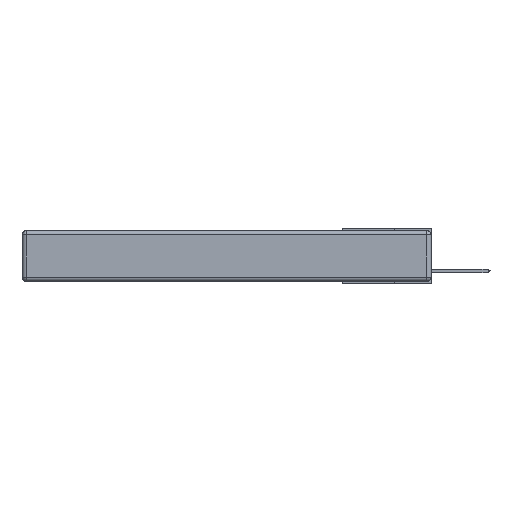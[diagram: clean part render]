
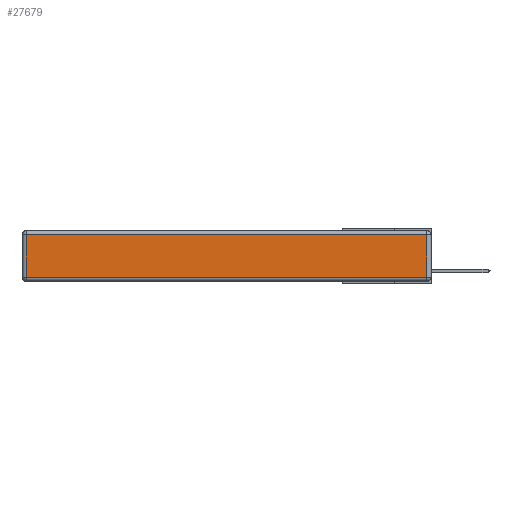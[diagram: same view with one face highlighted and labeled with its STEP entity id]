
A CAD part, left-side view. The second image highlights one B-rep face of the part: STEP entity #27679.
In plain terms, the highlighted planar face has unit normal (-1, 0, 0).
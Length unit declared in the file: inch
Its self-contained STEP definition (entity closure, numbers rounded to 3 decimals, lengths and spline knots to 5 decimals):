
#69 = DIRECTION ( 'NONE',  ( 0., 0., -1. ) ) ;
#555 = VECTOR ( 'NONE', #26867, 39.37008 ) ;
#1219 = VERTEX_POINT ( 'NONE', #25507 ) ;
#1252 = PLANE ( 'NONE',  #25136 ) ;
#1460 = DIRECTION ( 'NONE',  ( -1., 0., 0. ) ) ;
#2239 = VERTEX_POINT ( 'NONE', #18584 ) ;
#2263 = CARTESIAN_POINT ( 'NONE',  ( 0., 0., -0.313 ) ) ;
#2617 = ORIENTED_EDGE ( 'NONE', *, *, #20545, .T. ) ;
#3060 = ORIENTED_EDGE ( 'NONE', *, *, #13140, .T. ) ;
#3183 = CARTESIAN_POINT ( 'NONE',  ( 0., 0., -0.343 ) ) ;
#4995 = CARTESIAN_POINT ( 'NONE',  ( 0., 2.72, -0.343 ) ) ;
#6044 = CARTESIAN_POINT ( 'NONE',  ( 0., 2.75, -0.03 ) ) ;
#6498 = DIRECTION ( 'NONE',  ( 0., 0., 1. ) ) ;
#7588 = EDGE_CURVE ( 'NONE', #2239, #1219, #19691, .T. ) ;
#7644 = DIRECTION ( 'NONE',  ( 0., 0., 1. ) ) ;
#8942 = EDGE_CURVE ( 'NONE', #30396, #2239, #10089, .T. ) ;
#9676 = ORIENTED_EDGE ( 'NONE', *, *, #7588, .T. ) ;
#10089 = LINE ( 'NONE', #2263, #555 ) ;
#12495 = VECTOR ( 'NONE', #69, 39.37008 ) ;
#13140 = EDGE_CURVE ( 'NONE', #24433, #30396, #26180, .T. ) ;
#14855 = CARTESIAN_POINT ( 'NONE',  ( 0., 0.03, -0.343 ) ) ;
#15329 = FACE_OUTER_BOUND ( 'NONE', #15838, .T. ) ;
#15838 = EDGE_LOOP ( 'NONE', ( #23708, #9676, #2617, #3060 ) ) ;
#18584 = CARTESIAN_POINT ( 'NONE',  ( 0., 0.03, -0.313 ) ) ;
#19691 = LINE ( 'NONE', #14855, #20078 ) ;
#20078 = VECTOR ( 'NONE', #7644, 39.37008 ) ;
#20545 = EDGE_CURVE ( 'NONE', #1219, #24433, #22222, .T. ) ;
#21069 = VECTOR ( 'NONE', #21180, 39.37008 ) ;
#21118 = CARTESIAN_POINT ( 'NONE',  ( 0., 2.72, -0.313 ) ) ;
#21180 = DIRECTION ( 'NONE',  ( 0., 1., 0. ) ) ;
#22222 = LINE ( 'NONE', #6044, #21069 ) ;
#23708 = ORIENTED_EDGE ( 'NONE', *, *, #8942, .T. ) ;
#24433 = VERTEX_POINT ( 'NONE', #27270 ) ;
#25136 = AXIS2_PLACEMENT_3D ( 'NONE', #3183, #1460, #6498 ) ;
#25507 = CARTESIAN_POINT ( 'NONE',  ( 0., 0.03, -0.03 ) ) ;
#26180 = LINE ( 'NONE', #4995, #12495 ) ;
#26867 = DIRECTION ( 'NONE',  ( 0., -1., 0. ) ) ;
#27270 = CARTESIAN_POINT ( 'NONE',  ( 0., 2.72, -0.03 ) ) ;
#27679 = ADVANCED_FACE ( 'NONE', ( #15329 ), #1252, .T. ) ;
#30396 = VERTEX_POINT ( 'NONE', #21118 ) ;
